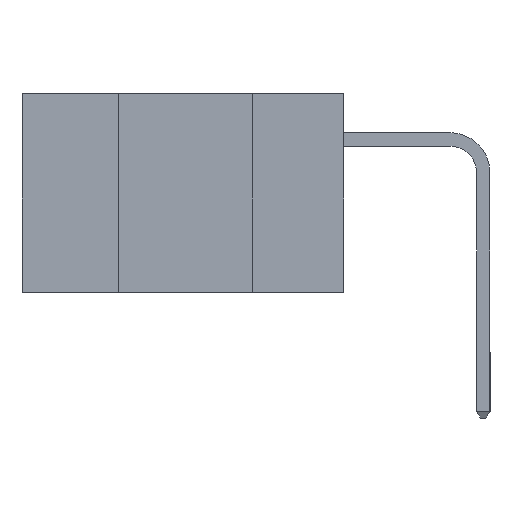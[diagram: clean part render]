
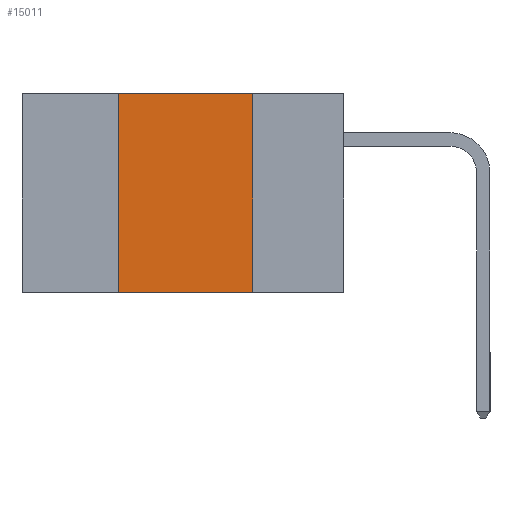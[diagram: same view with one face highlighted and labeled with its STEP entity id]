
A CAD part, left-side view. The second image highlights one B-rep face of the part: STEP entity #15011.
In plain terms, the highlighted planar face has unit normal (-1, 0, 0).
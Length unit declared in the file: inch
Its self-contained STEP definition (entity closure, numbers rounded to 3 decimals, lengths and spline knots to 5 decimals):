
#257 = VECTOR ( 'NONE', #21014, 39.37008 ) ;
#395 = CARTESIAN_POINT ( 'NONE',  ( 0., 0.17, -0.37 ) ) ;
#945 = LINE ( 'NONE', #5635, #257 ) ;
#1368 = VECTOR ( 'NONE', #5469, 39.37008 ) ;
#5469 = DIRECTION ( 'NONE',  ( 0., -1., 0. ) ) ;
#5635 = CARTESIAN_POINT ( 'NONE',  ( 0., 0.42, 0. ) ) ;
#7079 = CARTESIAN_POINT ( 'NONE',  ( 0., 0.42, 0. ) ) ;
#7206 = EDGE_CURVE ( 'NONE', #22509, #12858, #945, .T. ) ;
#8451 = EDGE_CURVE ( 'NONE', #12858, #20142, #18452, .T. ) ;
#8658 = PLANE ( 'NONE',  #15960 ) ;
#8752 = CARTESIAN_POINT ( 'NONE',  ( 0., 0.6, 0. ) ) ;
#10940 = VERTEX_POINT ( 'NONE', #395 ) ;
#11078 = EDGE_LOOP ( 'NONE', ( #13960, #17538, #27629, #12530 ) ) ;
#12349 = EDGE_CURVE ( 'NONE', #20142, #10940, #26071, .T. ) ;
#12530 = ORIENTED_EDGE ( 'NONE', *, *, #12738, .T. ) ;
#12738 = EDGE_CURVE ( 'NONE', #22509, #10940, #23254, .T. ) ;
#12858 = VERTEX_POINT ( 'NONE', #7079 ) ;
#13960 = ORIENTED_EDGE ( 'NONE', *, *, #12349, .F. ) ;
#14116 = CARTESIAN_POINT ( 'NONE',  ( 0., 0.42, -0.37 ) ) ;
#15011 = ADVANCED_FACE ( 'NONE', ( #21579 ), #8658, .F. ) ;
#15156 = CARTESIAN_POINT ( 'NONE',  ( 0., 0.6, 0. ) ) ;
#15960 = AXIS2_PLACEMENT_3D ( 'NONE', #8752, #23997, #28248 ) ;
#16248 = DIRECTION ( 'NONE',  ( 0., -1., 0. ) ) ;
#17538 = ORIENTED_EDGE ( 'NONE', *, *, #8451, .F. ) ;
#18452 = LINE ( 'NONE', #15156, #22877 ) ;
#18458 = CARTESIAN_POINT ( 'NONE',  ( 0., 0.6, -0.37 ) ) ;
#20142 = VERTEX_POINT ( 'NONE', #28375 ) ;
#20926 = VECTOR ( 'NONE', #25453, 39.37008 ) ;
#21014 = DIRECTION ( 'NONE',  ( 0., 0., 1. ) ) ;
#21579 = FACE_OUTER_BOUND ( 'NONE', #11078, .T. ) ;
#22509 = VERTEX_POINT ( 'NONE', #14116 ) ;
#22877 = VECTOR ( 'NONE', #16248, 39.37008 ) ;
#23254 = LINE ( 'NONE', #18458, #1368 ) ;
#23997 = DIRECTION ( 'NONE',  ( 1., 0., 0. ) ) ;
#25453 = DIRECTION ( 'NONE',  ( 0., 0., -1. ) ) ;
#26071 = LINE ( 'NONE', #27562, #20926 ) ;
#27562 = CARTESIAN_POINT ( 'NONE',  ( 0., 0.17, 0. ) ) ;
#27629 = ORIENTED_EDGE ( 'NONE', *, *, #7206, .F. ) ;
#28248 = DIRECTION ( 'NONE',  ( 0., 0., -1. ) ) ;
#28375 = CARTESIAN_POINT ( 'NONE',  ( 0., 0.17, 0. ) ) ;
